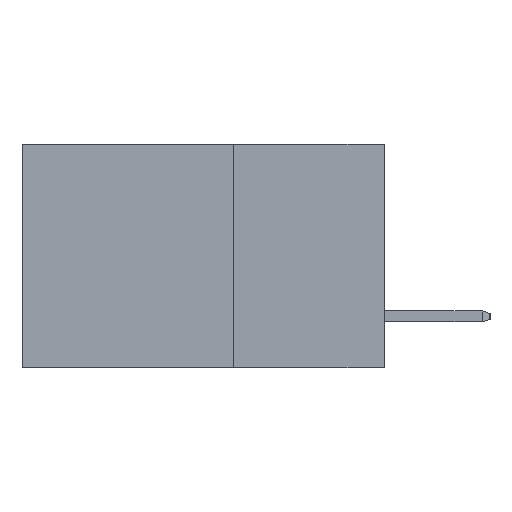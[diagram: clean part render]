
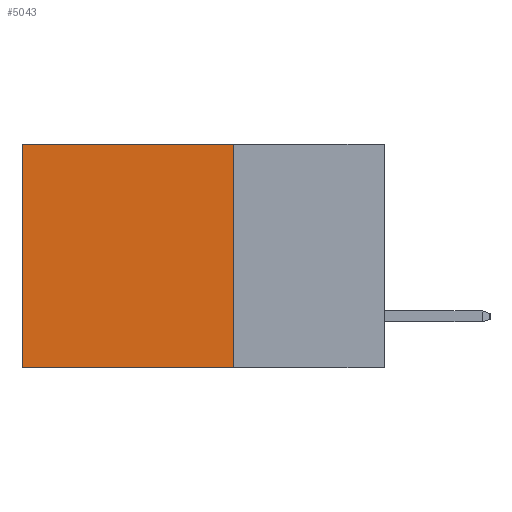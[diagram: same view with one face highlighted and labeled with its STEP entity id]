
A CAD part, left-side view. The second image highlights one B-rep face of the part: STEP entity #5043.
In plain terms, the highlighted planar face has unit normal (-1, 0, 0).
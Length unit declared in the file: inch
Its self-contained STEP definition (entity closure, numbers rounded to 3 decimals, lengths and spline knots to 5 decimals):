
#49 = ORIENTED_EDGE ( 'NONE', *, *, #9550, .F. ) ;
#80 = DIRECTION ( 'NONE',  ( 0., 0., -1. ) ) ;
#321 = ORIENTED_EDGE ( 'NONE', *, *, #5545, .T. ) ;
#752 = DIRECTION ( 'NONE',  ( 0., 0., -1. ) ) ;
#858 = CARTESIAN_POINT ( 'NONE',  ( 0.2615, 0.25, 0. ) ) ;
#909 = VERTEX_POINT ( 'NONE', #6420 ) ;
#1036 = DIRECTION ( 'NONE',  ( 0., 1., 0. ) ) ;
#2078 = LINE ( 'NONE', #9855, #8313 ) ;
#2800 = DIRECTION ( 'NONE',  ( 0., 0., -1. ) ) ;
#2971 = LINE ( 'NONE', #7628, #7047 ) ;
#3493 = CARTESIAN_POINT ( 'NONE',  ( 0.2615, 0.25, 0. ) ) ;
#4067 = EDGE_CURVE ( 'NONE', #5367, #5361, #2078, .T. ) ;
#4099 = EDGE_CURVE ( 'NONE', #5367, #909, #10139, .T. ) ;
#4446 = CARTESIAN_POINT ( 'NONE',  ( 0.2615, 0.6, -0.37 ) ) ;
#4635 = LINE ( 'NONE', #4446, #6515 ) ;
#4739 = ORIENTED_EDGE ( 'NONE', *, *, #4099, .T. ) ;
#4842 = AXIS2_PLACEMENT_3D ( 'NONE', #8924, #5745, #752 ) ;
#4898 = PLANE ( 'NONE',  #4842 ) ;
#5043 = ADVANCED_FACE ( 'NONE', ( #5142 ), #4898, .F. ) ;
#5142 = FACE_OUTER_BOUND ( 'NONE', #7475, .T. ) ;
#5361 = VERTEX_POINT ( 'NONE', #8252 ) ;
#5367 = VERTEX_POINT ( 'NONE', #858 ) ;
#5545 = EDGE_CURVE ( 'NONE', #909, #6985, #4635, .T. ) ;
#5745 = DIRECTION ( 'NONE',  ( 1., 0., 0. ) ) ;
#6420 = CARTESIAN_POINT ( 'NONE',  ( 0.2615, 0.6, 0. ) ) ;
#6515 = VECTOR ( 'NONE', #2800, 39.37008 ) ;
#6626 = ORIENTED_EDGE ( 'NONE', *, *, #4067, .F. ) ;
#6985 = VERTEX_POINT ( 'NONE', #10371 ) ;
#7047 = VECTOR ( 'NONE', #1036, 39.37008 ) ;
#7475 = EDGE_LOOP ( 'NONE', ( #321, #49, #6626, #4739 ) ) ;
#7628 = CARTESIAN_POINT ( 'NONE',  ( 0.2615, 0.25, -0.37 ) ) ;
#8252 = CARTESIAN_POINT ( 'NONE',  ( 0.2615, 0.25, -0.37 ) ) ;
#8313 = VECTOR ( 'NONE', #80, 39.37008 ) ;
#8329 = DIRECTION ( 'NONE',  ( 0., 1., 0. ) ) ;
#8924 = CARTESIAN_POINT ( 'NONE',  ( 0.2615, 0.25, -0.37 ) ) ;
#9550 = EDGE_CURVE ( 'NONE', #5361, #6985, #2971, .T. ) ;
#9855 = CARTESIAN_POINT ( 'NONE',  ( 0.2615, 0.25, -0.37 ) ) ;
#10139 = LINE ( 'NONE', #3493, #10386 ) ;
#10371 = CARTESIAN_POINT ( 'NONE',  ( 0.2615, 0.6, -0.37 ) ) ;
#10386 = VECTOR ( 'NONE', #8329, 39.37008 ) ;
